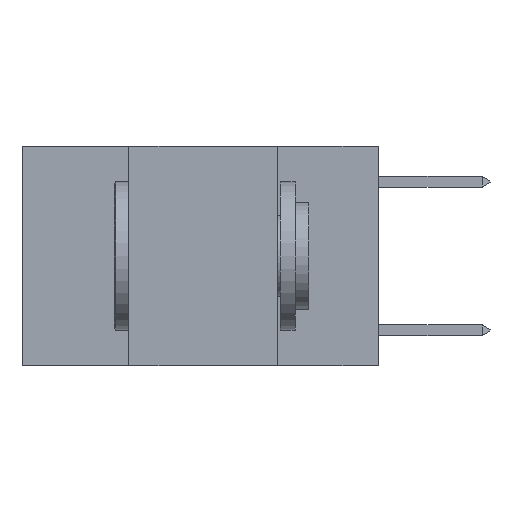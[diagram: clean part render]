
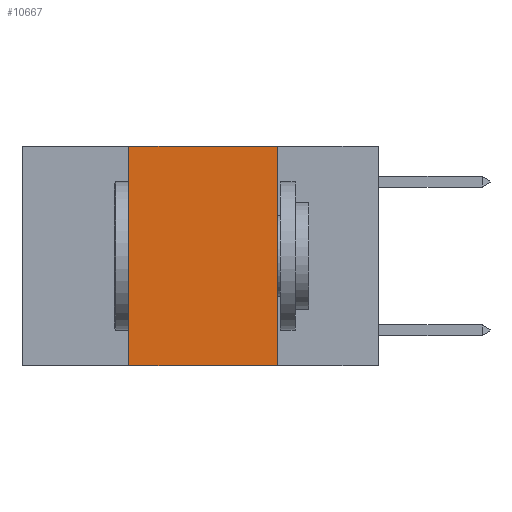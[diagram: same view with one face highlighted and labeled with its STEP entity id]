
A CAD part, left-side view. The second image highlights one B-rep face of the part: STEP entity #10667.
In plain terms, the highlighted planar face has unit normal (-1, 0, 0).
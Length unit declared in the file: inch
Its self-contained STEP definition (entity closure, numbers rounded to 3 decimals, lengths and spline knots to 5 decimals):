
#1299 = VECTOR ( 'NONE', #12289, 39.37008 ) ;
#1474 = VECTOR ( 'NONE', #20998, 39.37008 ) ;
#3123 = LINE ( 'NONE', #21796, #9832 ) ;
#3539 = EDGE_CURVE ( 'NONE', #22179, #6957, #10763, .T. ) ;
#3600 = VERTEX_POINT ( 'NONE', #15155 ) ;
#4679 = EDGE_CURVE ( 'NONE', #3600, #6957, #23448, .T. ) ;
#5145 = CARTESIAN_POINT ( 'NONE',  ( 0., 0.42, 0. ) ) ;
#5216 = DIRECTION ( 'NONE',  ( 0., 0., -1. ) ) ;
#6957 = VERTEX_POINT ( 'NONE', #22600 ) ;
#8332 = CARTESIAN_POINT ( 'NONE',  ( 0., 0.17, 0. ) ) ;
#8986 = FACE_OUTER_BOUND ( 'NONE', #23502, .T. ) ;
#9674 = ORIENTED_EDGE ( 'NONE', *, *, #10627, .F. ) ;
#9740 = ORIENTED_EDGE ( 'NONE', *, *, #4679, .T. ) ;
#9832 = VECTOR ( 'NONE', #18354, 39.37008 ) ;
#10398 = CARTESIAN_POINT ( 'NONE',  ( 0., 0.6, -0.37 ) ) ;
#10627 = EDGE_CURVE ( 'NONE', #17074, #22179, #21559, .T. ) ;
#10667 = ADVANCED_FACE ( 'NONE', ( #8986 ), #21915, .F. ) ;
#10763 = LINE ( 'NONE', #13202, #1474 ) ;
#10938 = CARTESIAN_POINT ( 'NONE',  ( 0., 0.6, 0. ) ) ;
#11710 = ORIENTED_EDGE ( 'NONE', *, *, #3539, .F. ) ;
#12128 = ORIENTED_EDGE ( 'NONE', *, *, #18898, .F. ) ;
#12289 = DIRECTION ( 'NONE',  ( 0., -1., 0. ) ) ;
#13202 = CARTESIAN_POINT ( 'NONE',  ( 0., 0.17, 0. ) ) ;
#14370 = DIRECTION ( 'NONE',  ( 1., 0., 0. ) ) ;
#14947 = AXIS2_PLACEMENT_3D ( 'NONE', #10938, #14370, #5216 ) ;
#15155 = CARTESIAN_POINT ( 'NONE',  ( 0., 0.42, -0.37 ) ) ;
#17074 = VERTEX_POINT ( 'NONE', #5145 ) ;
#17940 = DIRECTION ( 'NONE',  ( 0., -1., 0. ) ) ;
#18354 = DIRECTION ( 'NONE',  ( 0., 0., 1. ) ) ;
#18583 = VECTOR ( 'NONE', #17940, 39.37008 ) ;
#18898 = EDGE_CURVE ( 'NONE', #3600, #17074, #3123, .T. ) ;
#20998 = DIRECTION ( 'NONE',  ( 0., 0., -1. ) ) ;
#21559 = LINE ( 'NONE', #23865, #1299 ) ;
#21796 = CARTESIAN_POINT ( 'NONE',  ( 0., 0.42, 0. ) ) ;
#21915 = PLANE ( 'NONE',  #14947 ) ;
#22179 = VERTEX_POINT ( 'NONE', #8332 ) ;
#22600 = CARTESIAN_POINT ( 'NONE',  ( 0., 0.17, -0.37 ) ) ;
#23448 = LINE ( 'NONE', #10398, #18583 ) ;
#23502 = EDGE_LOOP ( 'NONE', ( #11710, #9674, #12128, #9740 ) ) ;
#23865 = CARTESIAN_POINT ( 'NONE',  ( 0., 0.6, 0. ) ) ;
